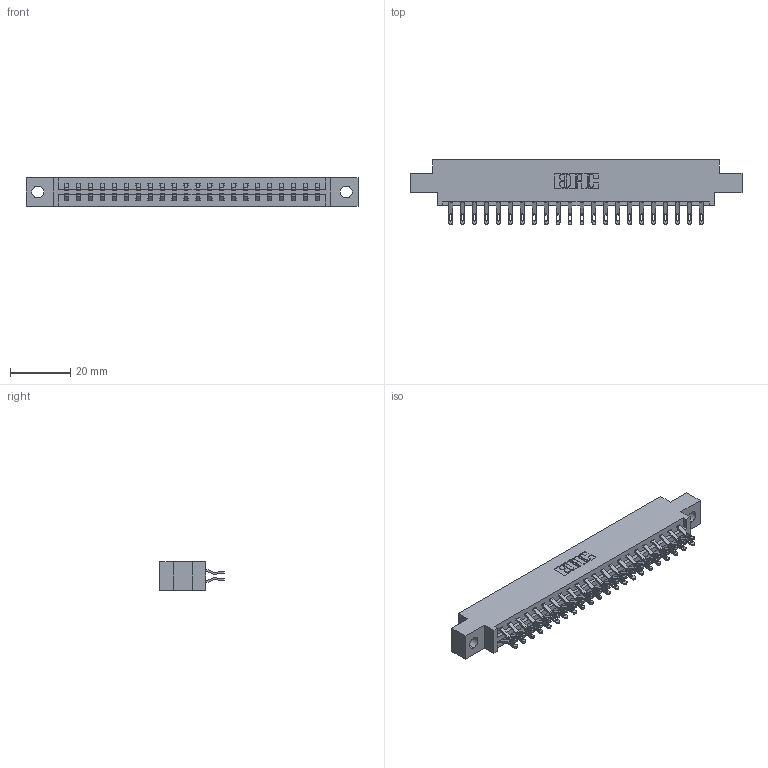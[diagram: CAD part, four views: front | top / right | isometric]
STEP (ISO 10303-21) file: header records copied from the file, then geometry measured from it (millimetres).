
FILE_DESCRIPTION (( 'STEP AP203' ), '1' );
FILE_NAME ('337-044-555-804.STEP', '2018-08-09T05:45:02', ( '' ), ( '' ), 'SwSTEP 2.0', 'SolidWorks 2016', '' );
FILE_SCHEMA (( 'CONFIG_CONTROL_DESIGN' ));
Length unit declared in the file: inch
Products named in the file (3): 337 Part_0.170 Offset - 0.156 Dia-TH; 345-292-001_555 Tail; 337-044-555-804
Assembly tree (45 placements, depth 2):
  337-044-555-804
    337 Part_0.170 Offset - 0.156 Dia-TH
    345-292-001_555 Tail  x44
Bounding box: 110.19 x 21.47 x 9.4 mm (x, y, z)
Volume: 11268.2 mm3; surface area: 12930.7 mm2
Topology: 45 solids, 45 shells, 2758 faces, 8639 edges, 5758 vertices
Faces by surface type: plane 1658, cylinder 1100
Entity records: 20105 total; most frequent: CARTESIAN_POINT 3440, ORIENTED_EDGE 3346, DIRECTION 2933, EDGE_CURVE 1673, VECTOR 1525, LINE 1525, VERTEX_POINT 1114, AXIS2_PLACEMENT_3D 704
